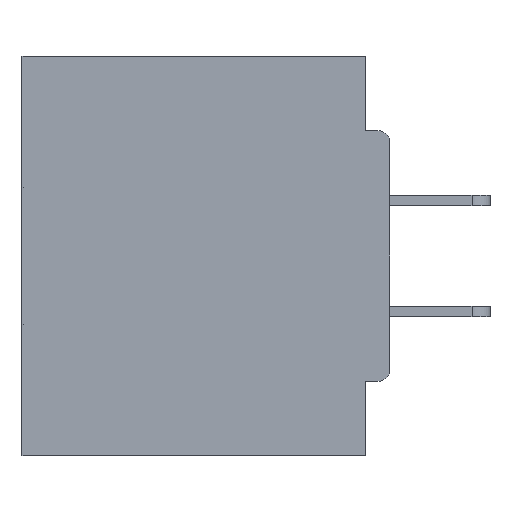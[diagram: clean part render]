
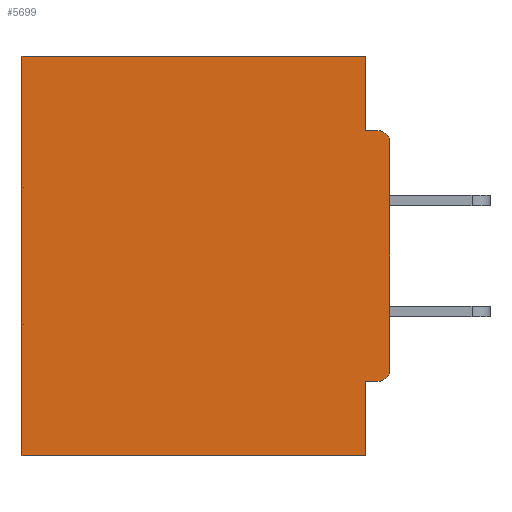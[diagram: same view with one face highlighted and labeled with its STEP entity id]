
A CAD part, left-side view. The second image highlights one B-rep face of the part: STEP entity #5699.
In plain terms, the highlighted planar face has unit normal (-1, 0, 0).
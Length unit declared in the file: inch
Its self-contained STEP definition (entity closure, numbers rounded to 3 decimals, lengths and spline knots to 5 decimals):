
#978 = VECTOR ( 'NONE', #20075, 39.37008 ) ;
#1410 = VECTOR ( 'NONE', #22493, 39.37008 ) ;
#1515 = EDGE_LOOP ( 'NONE', ( #11314, #15931, #22248, #7921, #35299, #26023, #28181, #1671, #15857, #11987 ) ) ;
#1671 = ORIENTED_EDGE ( 'NONE', *, *, #7399, .F. ) ;
#3114 = DIRECTION ( 'NONE',  ( 0., 0., -1. ) ) ;
#3209 = CARTESIAN_POINT ( 'NONE',  ( 0.298, 0.031, 0. ) ) ;
#3356 = CARTESIAN_POINT ( 'NONE',  ( 0.298, 0., -0.0935 ) ) ;
#3496 = DIRECTION ( 'NONE',  ( 0., -1., 0. ) ) ;
#3625 = LINE ( 'NONE', #9437, #6484 ) ;
#3931 = CIRCLE ( 'NONE', #14088, 0.015 ) ;
#4694 = CIRCLE ( 'NONE', #39343, 0.015 ) ;
#5324 = CARTESIAN_POINT ( 'NONE',  ( 0.298, 0.46, 0. ) ) ;
#5327 = VERTEX_POINT ( 'NONE', #5657 ) ;
#5657 = CARTESIAN_POINT ( 'NONE',  ( 0.298, 0.031, -0.0935 ) ) ;
#5699 = ADVANCED_FACE ( 'NONE', ( #11840 ), #18814, .F. ) ;
#5851 = LINE ( 'NONE', #38558, #978 ) ;
#6484 = VECTOR ( 'NONE', #12267, 39.37008 ) ;
#6874 = CARTESIAN_POINT ( 'NONE',  ( 0.298, 0., 0. ) ) ;
#7126 = CARTESIAN_POINT ( 'NONE',  ( 0.298, 0.031, -0.5 ) ) ;
#7399 = EDGE_CURVE ( 'NONE', #22430, #13316, #5851, .T. ) ;
#7866 = DIRECTION ( 'NONE',  ( -1., 0., 0. ) ) ;
#7921 = ORIENTED_EDGE ( 'NONE', *, *, #25000, .T. ) ;
#8678 = CARTESIAN_POINT ( 'NONE',  ( 0.298, 0.015, -0.3915 ) ) ;
#9437 = CARTESIAN_POINT ( 'NONE',  ( 0.298, 0.46, 0. ) ) ;
#9456 = DIRECTION ( 'NONE',  ( 0., 0., -1. ) ) ;
#10171 = CARTESIAN_POINT ( 'NONE',  ( 0.298, 0.015, -0.0935 ) ) ;
#11314 = ORIENTED_EDGE ( 'NONE', *, *, #30505, .T. ) ;
#11840 = FACE_OUTER_BOUND ( 'NONE', #1515, .T. ) ;
#11987 = ORIENTED_EDGE ( 'NONE', *, *, #35387, .F. ) ;
#12267 = DIRECTION ( 'NONE',  ( 0., 0., -1. ) ) ;
#12299 = EDGE_CURVE ( 'NONE', #25524, #27027, #3625, .T. ) ;
#12931 = CARTESIAN_POINT ( 'NONE',  ( 0.298, 0., -0.5 ) ) ;
#12948 = CARTESIAN_POINT ( 'NONE',  ( 0.298, 0., -0.3915 ) ) ;
#13030 = LINE ( 'NONE', #38093, #35363 ) ;
#13316 = VERTEX_POINT ( 'NONE', #36582 ) ;
#13603 = LINE ( 'NONE', #37194, #35470 ) ;
#14046 = LINE ( 'NONE', #12931, #28605 ) ;
#14088 = AXIS2_PLACEMENT_3D ( 'NONE', #8678, #22133, #21847 ) ;
#15855 = VERTEX_POINT ( 'NONE', #10171 ) ;
#15857 = ORIENTED_EDGE ( 'NONE', *, *, #21372, .T. ) ;
#15931 = ORIENTED_EDGE ( 'NONE', *, *, #37717, .F. ) ;
#16597 = DIRECTION ( 'NONE',  ( 0., 1., 0. ) ) ;
#17660 = VECTOR ( 'NONE', #25982, 39.37008 ) ;
#17992 = VERTEX_POINT ( 'NONE', #12948 ) ;
#18814 = PLANE ( 'NONE',  #23088 ) ;
#19213 = DIRECTION ( 'NONE',  ( 0., 0., -1. ) ) ;
#19640 = CARTESIAN_POINT ( 'NONE',  ( 0.298, 0.46, -0.5 ) ) ;
#20075 = DIRECTION ( 'NONE',  ( 0., 1., 0. ) ) ;
#20639 = DIRECTION ( 'NONE',  ( 0., 0., -1. ) ) ;
#21372 = EDGE_CURVE ( 'NONE', #22430, #17992, #3931, .T. ) ;
#21722 = EDGE_CURVE ( 'NONE', #26163, #27027, #14046, .T. ) ;
#21847 = DIRECTION ( 'NONE',  ( 0., 0., -1. ) ) ;
#22133 = DIRECTION ( 'NONE',  ( -1., 0., 0. ) ) ;
#22248 = ORIENTED_EDGE ( 'NONE', *, *, #34094, .F. ) ;
#22430 = VERTEX_POINT ( 'NONE', #38376 ) ;
#22493 = DIRECTION ( 'NONE',  ( 0., 0., -1. ) ) ;
#23088 = AXIS2_PLACEMENT_3D ( 'NONE', #37006, #24609, #9456 ) ;
#24609 = DIRECTION ( 'NONE',  ( 1., 0., 0. ) ) ;
#25000 = EDGE_CURVE ( 'NONE', #39023, #25524, #25879, .T. ) ;
#25524 = VERTEX_POINT ( 'NONE', #5324 ) ;
#25764 = LINE ( 'NONE', #3356, #39407 ) ;
#25879 = LINE ( 'NONE', #6874, #17660 ) ;
#25982 = DIRECTION ( 'NONE',  ( 0., 1., 0. ) ) ;
#26023 = ORIENTED_EDGE ( 'NONE', *, *, #21722, .F. ) ;
#26163 = VERTEX_POINT ( 'NONE', #33239 ) ;
#26439 = CARTESIAN_POINT ( 'NONE',  ( 0.298, 0.015, -0.1085 ) ) ;
#27027 = VERTEX_POINT ( 'NONE', #19640 ) ;
#28181 = ORIENTED_EDGE ( 'NONE', *, *, #38657, .F. ) ;
#28605 = VECTOR ( 'NONE', #16597, 39.37008 ) ;
#29082 = LINE ( 'NONE', #7126, #1410 ) ;
#30471 = CARTESIAN_POINT ( 'NONE',  ( 0.298, 0., -0.1085 ) ) ;
#30505 = EDGE_CURVE ( 'NONE', #32217, #15855, #4694, .T. ) ;
#32217 = VERTEX_POINT ( 'NONE', #30471 ) ;
#33239 = CARTESIAN_POINT ( 'NONE',  ( 0.298, 0.031, -0.5 ) ) ;
#34094 = EDGE_CURVE ( 'NONE', #39023, #5327, #13603, .T. ) ;
#35299 = ORIENTED_EDGE ( 'NONE', *, *, #12299, .T. ) ;
#35363 = VECTOR ( 'NONE', #19213, 39.37008 ) ;
#35387 = EDGE_CURVE ( 'NONE', #32217, #17992, #13030, .T. ) ;
#35470 = VECTOR ( 'NONE', #3114, 39.37008 ) ;
#36582 = CARTESIAN_POINT ( 'NONE',  ( 0.298, 0.031, -0.4065 ) ) ;
#37006 = CARTESIAN_POINT ( 'NONE',  ( 0.298, 0., 0. ) ) ;
#37194 = CARTESIAN_POINT ( 'NONE',  ( 0.298, 0.031, -0.5 ) ) ;
#37717 = EDGE_CURVE ( 'NONE', #5327, #15855, #25764, .T. ) ;
#38093 = CARTESIAN_POINT ( 'NONE',  ( 0.298, 0., 0. ) ) ;
#38376 = CARTESIAN_POINT ( 'NONE',  ( 0.298, 0.015, -0.4065 ) ) ;
#38558 = CARTESIAN_POINT ( 'NONE',  ( 0.298, 0., -0.4065 ) ) ;
#38657 = EDGE_CURVE ( 'NONE', #13316, #26163, #29082, .T. ) ;
#39023 = VERTEX_POINT ( 'NONE', #3209 ) ;
#39343 = AXIS2_PLACEMENT_3D ( 'NONE', #26439, #7866, #20639 ) ;
#39407 = VECTOR ( 'NONE', #3496, 39.37008 ) ;
